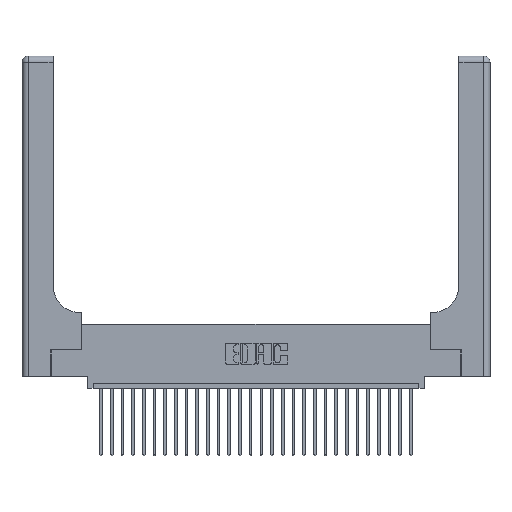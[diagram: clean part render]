
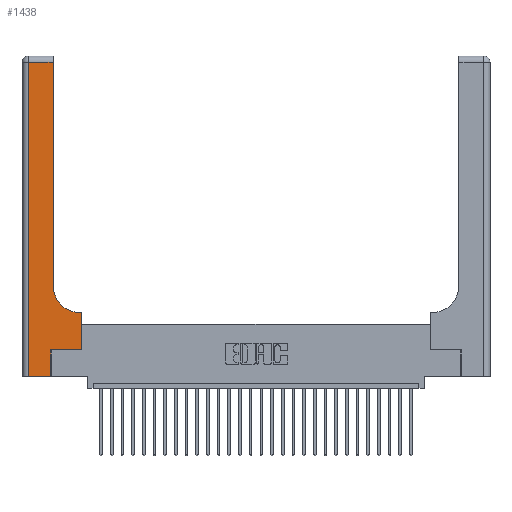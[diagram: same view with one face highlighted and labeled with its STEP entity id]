
A CAD part, top view. The second image highlights one B-rep face of the part: STEP entity #1438.
In plain terms, the highlighted planar face has unit normal (0, 0, 1).
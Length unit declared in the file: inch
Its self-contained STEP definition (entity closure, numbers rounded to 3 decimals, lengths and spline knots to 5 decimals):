
#132 = ORIENTED_EDGE ( 'NONE', *, *, #5614, .T. ) ;
#1156 = ORIENTED_EDGE ( 'NONE', *, *, #6771, .T. ) ;
#1438 = ADVANCED_FACE ( 'NONE', ( #3292 ), #15149, .F. ) ;
#1521 = VECTOR ( 'NONE', #5981, 39.37008 ) ;
#2427 = EDGE_CURVE ( 'NONE', #5042, #15770, #19648, .T. ) ;
#3139 = CARTESIAN_POINT ( 'NONE',  ( 0.2915, 2.94, 0.37 ) ) ;
#3292 = FACE_OUTER_BOUND ( 'NONE', #28600, .T. ) ;
#3683 = LINE ( 'NONE', #3785, #1521 ) ;
#3785 = CARTESIAN_POINT ( 'NONE',  ( 0.2915, 3., 0.37 ) ) ;
#4020 = ORIENTED_EDGE ( 'NONE', *, *, #2427, .T. ) ;
#4250 = LINE ( 'NONE', #19106, #21750 ) ;
#4326 = ORIENTED_EDGE ( 'NONE', *, *, #21659, .T. ) ;
#4802 = DIRECTION ( 'NONE',  ( -1., 0., 0. ) ) ;
#5042 = VERTEX_POINT ( 'NONE', #9013 ) ;
#5614 = EDGE_CURVE ( 'NONE', #9840, #5042, #15907, .T. ) ;
#5981 = DIRECTION ( 'NONE',  ( 0., 1., 0. ) ) ;
#6235 = VERTEX_POINT ( 'NONE', #14425 ) ;
#6333 = CARTESIAN_POINT ( 'NONE',  ( 0.06, 3., 0.37 ) ) ;
#6771 = EDGE_CURVE ( 'NONE', #14738, #9840, #3683, .T. ) ;
#6879 = CARTESIAN_POINT ( 'NONE',  ( 0.269, 0., 0.37 ) ) ;
#7433 = EDGE_CURVE ( 'NONE', #26083, #27161, #14714, .T. ) ;
#8386 = EDGE_CURVE ( 'NONE', #27841, #6235, #21804, .T. ) ;
#8558 = ORIENTED_EDGE ( 'NONE', *, *, #17654, .T. ) ;
#9013 = CARTESIAN_POINT ( 'NONE',  ( 0.06, 2.94, 0.37 ) ) ;
#9594 = DIRECTION ( 'NONE',  ( 0., 1., 0. ) ) ;
#9653 = VECTOR ( 'NONE', #14340, 39.37008 ) ;
#9840 = VERTEX_POINT ( 'NONE', #3139 ) ;
#9886 = ORIENTED_EDGE ( 'NONE', *, *, #14554, .T. ) ;
#10296 = VECTOR ( 'NONE', #25472, 39.37008 ) ;
#11344 = ORIENTED_EDGE ( 'NONE', *, *, #17421, .T. ) ;
#11711 = CARTESIAN_POINT ( 'NONE',  ( 0., 0., 0.37 ) ) ;
#11964 = LINE ( 'NONE', #23037, #27279 ) ;
#13287 = VECTOR ( 'NONE', #17312, 39.37008 ) ;
#14140 = ORIENTED_EDGE ( 'NONE', *, *, #8386, .T. ) ;
#14340 = DIRECTION ( 'NONE',  ( 0., -1., 0. ) ) ;
#14405 = CARTESIAN_POINT ( 'NONE',  ( 0.269, 0., 0.37 ) ) ;
#14425 = CARTESIAN_POINT ( 'NONE',  ( 0.269, 0.25, 0.37 ) ) ;
#14554 = EDGE_CURVE ( 'NONE', #27161, #18204, #11964, .T. ) ;
#14714 = LINE ( 'NONE', #21491, #13287 ) ;
#14738 = VERTEX_POINT ( 'NONE', #25716 ) ;
#14943 = CARTESIAN_POINT ( 'NONE',  ( 0., 3., 0.37 ) ) ;
#15149 = PLANE ( 'NONE',  #24000 ) ;
#15751 = VECTOR ( 'NONE', #9594, 39.37008 ) ;
#15770 = VERTEX_POINT ( 'NONE', #25919 ) ;
#15907 = LINE ( 'NONE', #29339, #27291 ) ;
#16049 = DIRECTION ( 'NONE',  ( -1., 0., 0. ) ) ;
#17312 = DIRECTION ( 'NONE',  ( 0., 1., 0. ) ) ;
#17421 = EDGE_CURVE ( 'NONE', #18204, #14738, #26035, .T. ) ;
#17479 = DIRECTION ( 'NONE',  ( -1., 0., 0. ) ) ;
#17654 = EDGE_CURVE ( 'NONE', #6235, #26083, #4250, .T. ) ;
#18204 = VERTEX_POINT ( 'NONE', #27667 ) ;
#19106 = CARTESIAN_POINT ( 'NONE',  ( 0.269, 0.25, 0.37 ) ) ;
#19648 = LINE ( 'NONE', #6333, #9653 ) ;
#20404 = CARTESIAN_POINT ( 'NONE',  ( 0.5415, 0.85, 0.37 ) ) ;
#21078 = CARTESIAN_POINT ( 'NONE',  ( 0.5585, 0.25, 0.37 ) ) ;
#21491 = CARTESIAN_POINT ( 'NONE',  ( 0.5585, 0.25, 0.37 ) ) ;
#21659 = EDGE_CURVE ( 'NONE', #15770, #27841, #22786, .T. ) ;
#21750 = VECTOR ( 'NONE', #27855, 39.37008 ) ;
#21804 = LINE ( 'NONE', #14405, #15751 ) ;
#22442 = DIRECTION ( 'NONE',  ( 1., 0., 0. ) ) ;
#22786 = LINE ( 'NONE', #11711, #10296 ) ;
#22826 = DIRECTION ( 'NONE',  ( 0., 0., -1. ) ) ;
#23037 = CARTESIAN_POINT ( 'NONE',  ( 0.2915, 0.6, 0.37 ) ) ;
#24000 = AXIS2_PLACEMENT_3D ( 'NONE', #14943, #26532, #17479 ) ;
#25472 = DIRECTION ( 'NONE',  ( 1., 0., 0. ) ) ;
#25716 = CARTESIAN_POINT ( 'NONE',  ( 0.2915, 0.85, 0.37 ) ) ;
#25919 = CARTESIAN_POINT ( 'NONE',  ( 0.06, 0., 0.37 ) ) ;
#26035 = CIRCLE ( 'NONE', #28810, 0.25 ) ;
#26083 = VERTEX_POINT ( 'NONE', #21078 ) ;
#26327 = ORIENTED_EDGE ( 'NONE', *, *, #7433, .T. ) ;
#26532 = DIRECTION ( 'NONE',  ( 0., 0., -1. ) ) ;
#27161 = VERTEX_POINT ( 'NONE', #27266 ) ;
#27266 = CARTESIAN_POINT ( 'NONE',  ( 0.5585, 0.6, 0.37 ) ) ;
#27279 = VECTOR ( 'NONE', #16049, 39.37008 ) ;
#27291 = VECTOR ( 'NONE', #4802, 39.37008 ) ;
#27667 = CARTESIAN_POINT ( 'NONE',  ( 0.5415, 0.6, 0.37 ) ) ;
#27841 = VERTEX_POINT ( 'NONE', #6879 ) ;
#27855 = DIRECTION ( 'NONE',  ( 1., 0., 0. ) ) ;
#28600 = EDGE_LOOP ( 'NONE', ( #1156, #132, #4020, #4326, #14140, #8558, #26327, #9886, #11344 ) ) ;
#28810 = AXIS2_PLACEMENT_3D ( 'NONE', #20404, #22826, #22442 ) ;
#29339 = CARTESIAN_POINT ( 'NONE',  ( 0., 2.94, 0.37 ) ) ;
